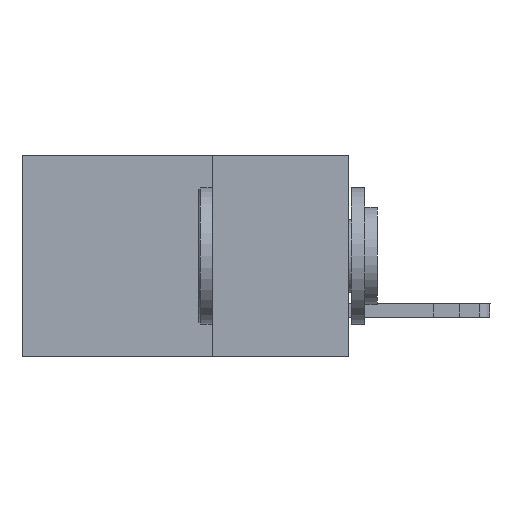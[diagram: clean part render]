
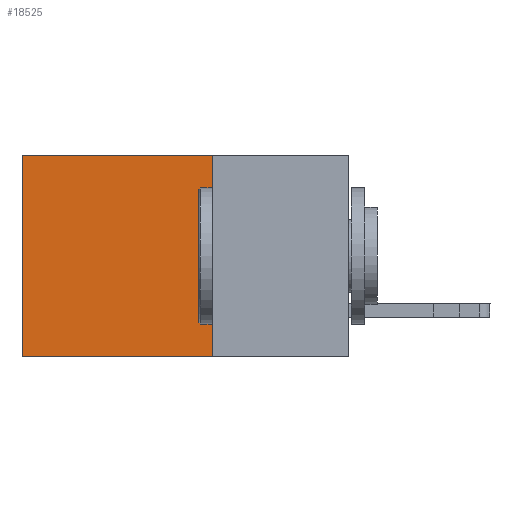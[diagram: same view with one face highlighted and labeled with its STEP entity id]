
A CAD part, left-side view. The second image highlights one B-rep face of the part: STEP entity #18525.
In plain terms, the highlighted planar face has unit normal (-1, 0, 0).
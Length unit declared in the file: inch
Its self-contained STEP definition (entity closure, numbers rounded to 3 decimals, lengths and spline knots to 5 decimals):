
#150 = CARTESIAN_POINT ( 'NONE',  ( 0.298, 0.25, -0.37 ) ) ;
#360 = VECTOR ( 'NONE', #4102, 39.37008 ) ;
#1237 = CARTESIAN_POINT ( 'NONE',  ( 0.298, 0.25, 0. ) ) ;
#1724 = VECTOR ( 'NONE', #12514, 39.37008 ) ;
#3879 = PLANE ( 'NONE',  #9341 ) ;
#4097 = DIRECTION ( 'NONE',  ( 0., 0., -1. ) ) ;
#4102 = DIRECTION ( 'NONE',  ( 0., 1., 0. ) ) ;
#4156 = CARTESIAN_POINT ( 'NONE',  ( 0.298, 0.25, 0. ) ) ;
#4477 = EDGE_CURVE ( 'NONE', #16780, #19597, #10522, .T. ) ;
#4988 = CARTESIAN_POINT ( 'NONE',  ( 0.298, 0.6, -0.37 ) ) ;
#6028 = LINE ( 'NONE', #15569, #360 ) ;
#6454 = EDGE_CURVE ( 'NONE', #19597, #6782, #12735, .T. ) ;
#6473 = ORIENTED_EDGE ( 'NONE', *, *, #9493, .T. ) ;
#6782 = VERTEX_POINT ( 'NONE', #4988 ) ;
#6824 = DIRECTION ( 'NONE',  ( 0., 0., -1. ) ) ;
#9341 = AXIS2_PLACEMENT_3D ( 'NONE', #4156, #15498, #4097 ) ;
#9347 = CARTESIAN_POINT ( 'NONE',  ( 0.298, 0.25, -0.37 ) ) ;
#9493 = EDGE_CURVE ( 'NONE', #12950, #6782, #17093, .T. ) ;
#10245 = FACE_OUTER_BOUND ( 'NONE', #18609, .T. ) ;
#10522 = LINE ( 'NONE', #14235, #1724 ) ;
#11148 = VECTOR ( 'NONE', #6824, 39.37008 ) ;
#11201 = VECTOR ( 'NONE', #13178, 39.37008 ) ;
#12514 = DIRECTION ( 'NONE',  ( 0., 0., -1. ) ) ;
#12735 = LINE ( 'NONE', #150, #11201 ) ;
#12950 = VERTEX_POINT ( 'NONE', #16933 ) ;
#13178 = DIRECTION ( 'NONE',  ( 0., 1., 0. ) ) ;
#14235 = CARTESIAN_POINT ( 'NONE',  ( 0.298, 0.25, 0. ) ) ;
#15354 = ORIENTED_EDGE ( 'NONE', *, *, #6454, .F. ) ;
#15498 = DIRECTION ( 'NONE',  ( 1., 0., 0. ) ) ;
#15569 = CARTESIAN_POINT ( 'NONE',  ( 0.298, 0.25, 0. ) ) ;
#16027 = EDGE_CURVE ( 'NONE', #16780, #12950, #6028, .T. ) ;
#16718 = CARTESIAN_POINT ( 'NONE',  ( 0.298, 0.6, 0. ) ) ;
#16780 = VERTEX_POINT ( 'NONE', #1237 ) ;
#16933 = CARTESIAN_POINT ( 'NONE',  ( 0.298, 0.6, 0. ) ) ;
#17093 = LINE ( 'NONE', #16718, #11148 ) ;
#18525 = ADVANCED_FACE ( 'NONE', ( #10245 ), #3879, .F. ) ;
#18609 = EDGE_LOOP ( 'NONE', ( #6473, #15354, #19006, #19050 ) ) ;
#19006 = ORIENTED_EDGE ( 'NONE', *, *, #4477, .F. ) ;
#19050 = ORIENTED_EDGE ( 'NONE', *, *, #16027, .T. ) ;
#19597 = VERTEX_POINT ( 'NONE', #9347 ) ;
